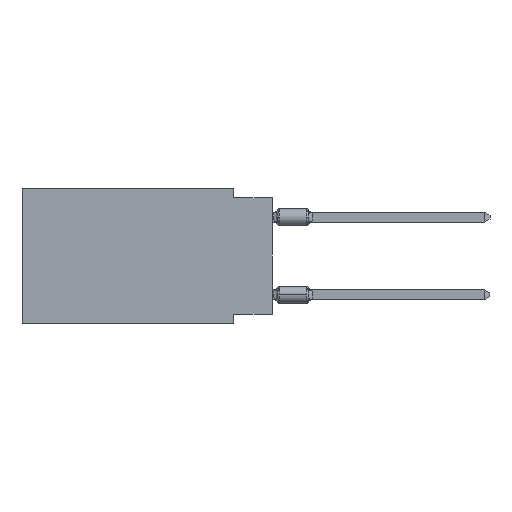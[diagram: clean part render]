
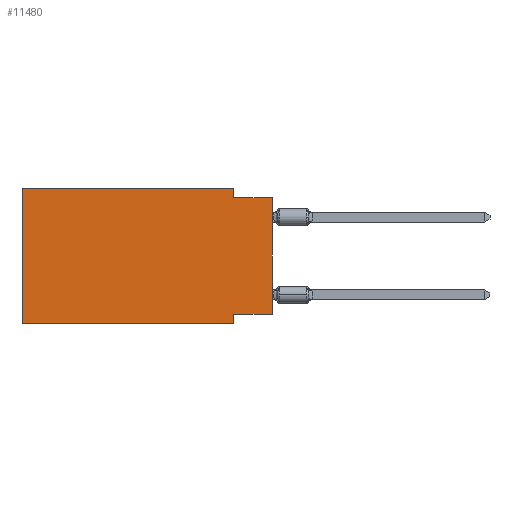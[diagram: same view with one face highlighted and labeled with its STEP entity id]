
A CAD part, left-side view. The second image highlights one B-rep face of the part: STEP entity #11480.
In plain terms, the highlighted planar face has unit normal (-1, 0, 0).
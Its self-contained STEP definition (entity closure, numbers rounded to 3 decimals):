
#59 = ORIENTED_EDGE ( 'NONE', *, *, #5701, .T. ) ;
#454 = DIRECTION ( 'NONE',  ( 0., 0., -1. ) ) ;
#762 = CARTESIAN_POINT ( 'NONE',  ( 0., 0., -8.255 ) ) ;
#1488 = VERTEX_POINT ( 'NONE', #3845 ) ;
#1690 = VERTEX_POINT ( 'NONE', #6579 ) ;
#1706 = EDGE_CURVE ( 'NONE', #10670, #1690, #4635, .T. ) ;
#1893 = EDGE_CURVE ( 'NONE', #8695, #5180, #6079, .T. ) ;
#2195 = PLANE ( 'NONE',  #5770 ) ;
#2377 = LINE ( 'NONE', #4423, #4886 ) ;
#2749 = VERTEX_POINT ( 'NONE', #9219 ) ;
#2753 = CARTESIAN_POINT ( 'NONE',  ( 0., 16.383, 0. ) ) ;
#2953 = DIRECTION ( 'NONE',  ( 0., 0., -1. ) ) ;
#3251 = CARTESIAN_POINT ( 'NONE',  ( 0., 0., -0.635 ) ) ;
#3425 = DIRECTION ( 'NONE',  ( 0., 0., 1. ) ) ;
#3503 = VERTEX_POINT ( 'NONE', #3251 ) ;
#3685 = ORIENTED_EDGE ( 'NONE', *, *, #1893, .F. ) ;
#3748 = EDGE_CURVE ( 'NONE', #1488, #10670, #10110, .T. ) ;
#3757 = CARTESIAN_POINT ( 'NONE',  ( 0., 2.54, -8.255 ) ) ;
#3845 = CARTESIAN_POINT ( 'NONE',  ( 0., 0., -8.255 ) ) ;
#4149 = LINE ( 'NONE', #8441, #10520 ) ;
#4252 = DIRECTION ( 'NONE',  ( 1., 0., 0. ) ) ;
#4383 = CARTESIAN_POINT ( 'NONE',  ( 0., 2.54, -0.635 ) ) ;
#4423 = CARTESIAN_POINT ( 'NONE',  ( 0., 0., -0.635 ) ) ;
#4497 = EDGE_CURVE ( 'NONE', #1488, #3503, #8588, .T. ) ;
#4635 = LINE ( 'NONE', #12931, #10611 ) ;
#4796 = VECTOR ( 'NONE', #5917, 1000. ) ;
#4886 = VECTOR ( 'NONE', #8650, 1000. ) ;
#4987 = ORIENTED_EDGE ( 'NONE', *, *, #6027, .F. ) ;
#5180 = VERTEX_POINT ( 'NONE', #4383 ) ;
#5411 = ORIENTED_EDGE ( 'NONE', *, *, #13335, .F. ) ;
#5548 = DIRECTION ( 'NONE',  ( 0., -1., 0. ) ) ;
#5701 = EDGE_CURVE ( 'NONE', #2749, #1690, #8927, .T. ) ;
#5770 = AXIS2_PLACEMENT_3D ( 'NONE', #6389, #4252, #2953 ) ;
#5880 = CARTESIAN_POINT ( 'NONE',  ( 0., 2.54, 0. ) ) ;
#5917 = DIRECTION ( 'NONE',  ( 0., 1., 0. ) ) ;
#6027 = EDGE_CURVE ( 'NONE', #11349, #8695, #4149, .T. ) ;
#6079 = LINE ( 'NONE', #5880, #6880 ) ;
#6136 = VECTOR ( 'NONE', #13259, 1000. ) ;
#6389 = CARTESIAN_POINT ( 'NONE',  ( 0., 16.383, 0. ) ) ;
#6579 = CARTESIAN_POINT ( 'NONE',  ( 0., 2.54, -8.89 ) ) ;
#6607 = EDGE_LOOP ( 'NONE', ( #9147, #5411, #3685, #4987, #7684, #59, #10727, #8727 ) ) ;
#6880 = VECTOR ( 'NONE', #12222, 1000. ) ;
#6960 = CARTESIAN_POINT ( 'NONE',  ( 0., 2.54, 0. ) ) ;
#7433 = FACE_OUTER_BOUND ( 'NONE', #6607, .T. ) ;
#7460 = EDGE_CURVE ( 'NONE', #2749, #11349, #13193, .T. ) ;
#7684 = ORIENTED_EDGE ( 'NONE', *, *, #7460, .F. ) ;
#7851 = VECTOR ( 'NONE', #3425, 1000. ) ;
#8441 = CARTESIAN_POINT ( 'NONE',  ( 0., 16.383, 0. ) ) ;
#8588 = LINE ( 'NONE', #12801, #7851 ) ;
#8650 = DIRECTION ( 'NONE',  ( 0., -1., 0. ) ) ;
#8663 = CARTESIAN_POINT ( 'NONE',  ( 0., 16.383, -8.89 ) ) ;
#8695 = VERTEX_POINT ( 'NONE', #6960 ) ;
#8727 = ORIENTED_EDGE ( 'NONE', *, *, #3748, .F. ) ;
#8927 = LINE ( 'NONE', #8663, #9618 ) ;
#9147 = ORIENTED_EDGE ( 'NONE', *, *, #4497, .T. ) ;
#9219 = CARTESIAN_POINT ( 'NONE',  ( 0., 16.383, -8.89 ) ) ;
#9239 = CARTESIAN_POINT ( 'NONE',  ( 0., 16.383, 0. ) ) ;
#9618 = VECTOR ( 'NONE', #5548, 1000. ) ;
#10110 = LINE ( 'NONE', #762, #4796 ) ;
#10520 = VECTOR ( 'NONE', #11544, 1000. ) ;
#10611 = VECTOR ( 'NONE', #454, 1000. ) ;
#10670 = VERTEX_POINT ( 'NONE', #3757 ) ;
#10727 = ORIENTED_EDGE ( 'NONE', *, *, #1706, .F. ) ;
#11349 = VERTEX_POINT ( 'NONE', #2753 ) ;
#11480 = ADVANCED_FACE ( 'NONE', ( #7433 ), #2195, .F. ) ;
#11544 = DIRECTION ( 'NONE',  ( 0., -1., 0. ) ) ;
#12222 = DIRECTION ( 'NONE',  ( 0., 0., -1. ) ) ;
#12801 = CARTESIAN_POINT ( 'NONE',  ( 0., 0., 0. ) ) ;
#12931 = CARTESIAN_POINT ( 'NONE',  ( 0., 2.54, -8.89 ) ) ;
#13193 = LINE ( 'NONE', #9239, #6136 ) ;
#13259 = DIRECTION ( 'NONE',  ( 0., 0., 1. ) ) ;
#13335 = EDGE_CURVE ( 'NONE', #5180, #3503, #2377, .T. ) ;
